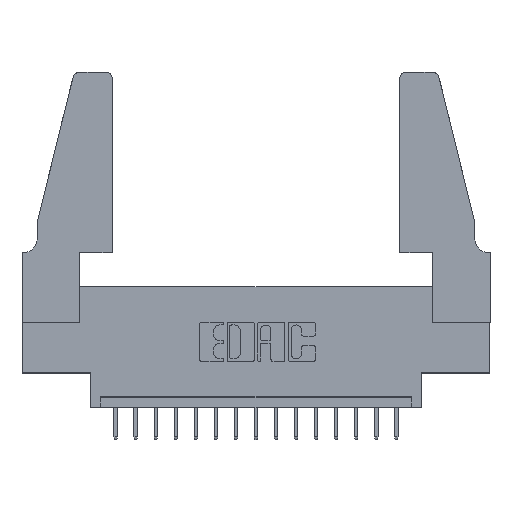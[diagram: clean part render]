
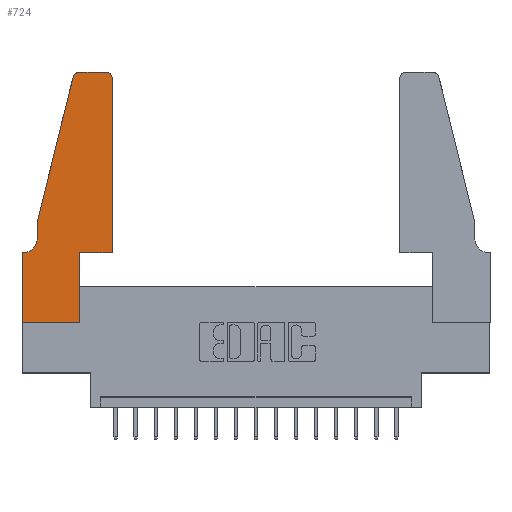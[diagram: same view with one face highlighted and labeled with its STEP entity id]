
A CAD part, top view. The second image highlights one B-rep face of the part: STEP entity #724.
In plain terms, the highlighted planar face has unit normal (0, 0, 1).
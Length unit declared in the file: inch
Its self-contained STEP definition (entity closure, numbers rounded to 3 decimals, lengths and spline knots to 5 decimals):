
#32 = DIRECTION ( 'NONE',  ( -1., 0., 0. ) ) ;
#184 = CARTESIAN_POINT ( 'NONE',  ( 0.4205, 1.22, 0.37 ) ) ;
#280 = EDGE_CURVE ( 'NONE', #10715, #3877, #2928, .T. ) ;
#518 = CIRCLE ( 'NONE', #15309, 0.03 ) ;
#724 = ADVANCED_FACE ( 'NONE', ( #2909 ), #16116, .T. ) ;
#1100 = LINE ( 'NONE', #13972, #2139 ) ;
#1184 = CARTESIAN_POINT ( 'NONE',  ( 0.0755, 0.42, 0.37 ) ) ;
#1493 = LINE ( 'NONE', #4410, #15894 ) ;
#1958 = LINE ( 'NONE', #9792, #9245 ) ;
#2072 = VERTEX_POINT ( 'NONE', #5516 ) ;
#2089 = VERTEX_POINT ( 'NONE', #15942 ) ;
#2139 = VECTOR ( 'NONE', #7368, 39.37008 ) ;
#2279 = VERTEX_POINT ( 'NONE', #9096 ) ;
#2305 = CIRCLE ( 'NONE', #2337, 0.07 ) ;
#2337 = AXIS2_PLACEMENT_3D ( 'NONE', #8147, #14754, #6668 ) ;
#2652 = ORIENTED_EDGE ( 'NONE', *, *, #280, .T. ) ;
#2909 = FACE_OUTER_BOUND ( 'NONE', #10358, .T. ) ;
#2928 = LINE ( 'NONE', #3397, #10830 ) ;
#2935 = CARTESIAN_POINT ( 'NONE',  ( 0.284, 1.22, 0.37 ) ) ;
#3004 = ORIENTED_EDGE ( 'NONE', *, *, #8551, .T. ) ;
#3063 = DIRECTION ( 'NONE',  ( 0., 0., 1. ) ) ;
#3265 = DIRECTION ( 'NONE',  ( -0.239, -0.971, 0. ) ) ;
#3389 = VERTEX_POINT ( 'NONE', #11815 ) ;
#3397 = CARTESIAN_POINT ( 'NONE',  ( 0.0755, 0.35, 0.37 ) ) ;
#3621 = ORIENTED_EDGE ( 'NONE', *, *, #13398, .T. ) ;
#3826 = CARTESIAN_POINT ( 'NONE',  ( 0.2865, 0.35, 0.37 ) ) ;
#3877 = VERTEX_POINT ( 'NONE', #9202 ) ;
#4011 = CARTESIAN_POINT ( 'NONE',  ( 0.2865, 0.35, 0.37 ) ) ;
#4410 = CARTESIAN_POINT ( 'NONE',  ( 0.4505, 0.35, 0.37 ) ) ;
#4414 = DIRECTION ( 'NONE',  ( 1., 0., 0. ) ) ;
#4660 = LINE ( 'NONE', #6557, #17150 ) ;
#4818 = CARTESIAN_POINT ( 'NONE',  ( 0.4505, 0.35, 0.37 ) ) ;
#5010 = CARTESIAN_POINT ( 'NONE',  ( 0.284, 1.25, 0.37 ) ) ;
#5516 = CARTESIAN_POINT ( 'NONE',  ( 0.25487, 1.22718, 0.37 ) ) ;
#5517 = CARTESIAN_POINT ( 'NONE',  ( 0.0755, 0.5, 0.37 ) ) ;
#5635 = DIRECTION ( 'NONE',  ( 0., 0., 1. ) ) ;
#5696 = DIRECTION ( 'NONE',  ( 1., 0., 0. ) ) ;
#5964 = EDGE_CURVE ( 'NONE', #11025, #10715, #2305, .T. ) ;
#6050 = ORIENTED_EDGE ( 'NONE', *, *, #5964, .T. ) ;
#6340 = VECTOR ( 'NONE', #15915, 39.37008 ) ;
#6557 = CARTESIAN_POINT ( 'NONE',  ( 0., 0., 0.37 ) ) ;
#6668 = DIRECTION ( 'NONE',  ( -1., 0., 0. ) ) ;
#6837 = EDGE_CURVE ( 'NONE', #3877, #2089, #4660, .T. ) ;
#7201 = AXIS2_PLACEMENT_3D ( 'NONE', #184, #3063, #4414 ) ;
#7368 = DIRECTION ( 'NONE',  ( 0., 1., 0. ) ) ;
#7453 = ORIENTED_EDGE ( 'NONE', *, *, #15161, .T. ) ;
#7460 = DIRECTION ( 'NONE',  ( -1., 0., 0. ) ) ;
#8147 = CARTESIAN_POINT ( 'NONE',  ( 0.0055, 0.42, 0.37 ) ) ;
#8551 = EDGE_CURVE ( 'NONE', #15216, #13591, #11642, .T. ) ;
#8632 = ORIENTED_EDGE ( 'NONE', *, *, #12052, .T. ) ;
#8824 = CARTESIAN_POINT ( 'NONE',  ( 0.4205, 1.25, 0.37 ) ) ;
#9096 = CARTESIAN_POINT ( 'NONE',  ( 0.4505, 1.22, 0.37 ) ) ;
#9129 = VECTOR ( 'NONE', #32, 39.37008 ) ;
#9179 = ORIENTED_EDGE ( 'NONE', *, *, #15856, .T. ) ;
#9202 = CARTESIAN_POINT ( 'NONE',  ( 0., 0.35, 0.37 ) ) ;
#9245 = VECTOR ( 'NONE', #3265, 39.37008 ) ;
#9792 = CARTESIAN_POINT ( 'NONE',  ( 0.0755, 0.5, 0.37 ) ) ;
#9909 = LINE ( 'NONE', #11866, #14104 ) ;
#10358 = EDGE_LOOP ( 'NONE', ( #3004, #7453, #9179, #14439, #6050, #2652, #10585, #3621, #8632, #16188, #12047, #15793 ) ) ;
#10585 = ORIENTED_EDGE ( 'NONE', *, *, #6837, .T. ) ;
#10599 = DIRECTION ( 'NONE',  ( 0., -1., 0. ) ) ;
#10715 = VERTEX_POINT ( 'NONE', #14547 ) ;
#10777 = DIRECTION ( 'NONE',  ( 1., 0., 0. ) ) ;
#10830 = VECTOR ( 'NONE', #7460, 39.37008 ) ;
#10996 = DIRECTION ( 'NONE',  ( 0., -1., 0. ) ) ;
#11025 = VERTEX_POINT ( 'NONE', #1184 ) ;
#11181 = EDGE_CURVE ( 'NONE', #2279, #15216, #12812, .T. ) ;
#11642 = LINE ( 'NONE', #12044, #9129 ) ;
#11815 = CARTESIAN_POINT ( 'NONE',  ( 0.2865, 0., 0.37 ) ) ;
#11866 = CARTESIAN_POINT ( 'NONE',  ( 0., 0., 0.37 ) ) ;
#11966 = DIRECTION ( 'NONE',  ( 0., 0., 1. ) ) ;
#12043 = DIRECTION ( 'NONE',  ( 1., 0., 0. ) ) ;
#12044 = CARTESIAN_POINT ( 'NONE',  ( 0.2605, 1.25, 0.37 ) ) ;
#12047 = ORIENTED_EDGE ( 'NONE', *, *, #12852, .T. ) ;
#12052 = EDGE_CURVE ( 'NONE', #3389, #12997, #14455, .T. ) ;
#12119 = LINE ( 'NONE', #5517, #13783 ) ;
#12485 = DIRECTION ( 'NONE',  ( 1., 0., 0. ) ) ;
#12812 = CIRCLE ( 'NONE', #7201, 0.03 ) ;
#12852 = EDGE_CURVE ( 'NONE', #17245, #2279, #1100, .T. ) ;
#12997 = VERTEX_POINT ( 'NONE', #4011 ) ;
#13189 = AXIS2_PLACEMENT_3D ( 'NONE', #17279, #11966, #10777 ) ;
#13398 = EDGE_CURVE ( 'NONE', #2089, #3389, #9909, .T. ) ;
#13591 = VERTEX_POINT ( 'NONE', #5010 ) ;
#13783 = VECTOR ( 'NONE', #10996, 39.37008 ) ;
#13972 = CARTESIAN_POINT ( 'NONE',  ( 0.4505, 0.35, 0.37 ) ) ;
#14104 = VECTOR ( 'NONE', #12043, 39.37008 ) ;
#14225 = VERTEX_POINT ( 'NONE', #17053 ) ;
#14439 = ORIENTED_EDGE ( 'NONE', *, *, #16573, .T. ) ;
#14455 = LINE ( 'NONE', #3826, #6340 ) ;
#14547 = CARTESIAN_POINT ( 'NONE',  ( 0.0055, 0.35, 0.37 ) ) ;
#14754 = DIRECTION ( 'NONE',  ( 0., 0., -1. ) ) ;
#15161 = EDGE_CURVE ( 'NONE', #13591, #2072, #518, .T. ) ;
#15216 = VERTEX_POINT ( 'NONE', #8824 ) ;
#15309 = AXIS2_PLACEMENT_3D ( 'NONE', #2935, #5635, #5696 ) ;
#15793 = ORIENTED_EDGE ( 'NONE', *, *, #11181, .T. ) ;
#15856 = EDGE_CURVE ( 'NONE', #2072, #14225, #1958, .T. ) ;
#15894 = VECTOR ( 'NONE', #12485, 39.37008 ) ;
#15915 = DIRECTION ( 'NONE',  ( 0., 1., 0. ) ) ;
#15942 = CARTESIAN_POINT ( 'NONE',  ( 0., 0., 0.37 ) ) ;
#16116 = PLANE ( 'NONE',  #13189 ) ;
#16188 = ORIENTED_EDGE ( 'NONE', *, *, #16936, .T. ) ;
#16573 = EDGE_CURVE ( 'NONE', #14225, #11025, #12119, .T. ) ;
#16936 = EDGE_CURVE ( 'NONE', #12997, #17245, #1493, .T. ) ;
#17053 = CARTESIAN_POINT ( 'NONE',  ( 0.0755, 0.5, 0.37 ) ) ;
#17150 = VECTOR ( 'NONE', #10599, 39.37008 ) ;
#17245 = VERTEX_POINT ( 'NONE', #4818 ) ;
#17279 = CARTESIAN_POINT ( 'NONE',  ( 0., 0.35, 0.37 ) ) ;
